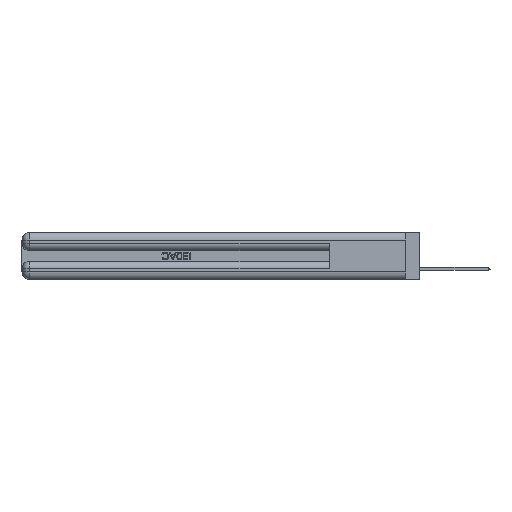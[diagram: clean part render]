
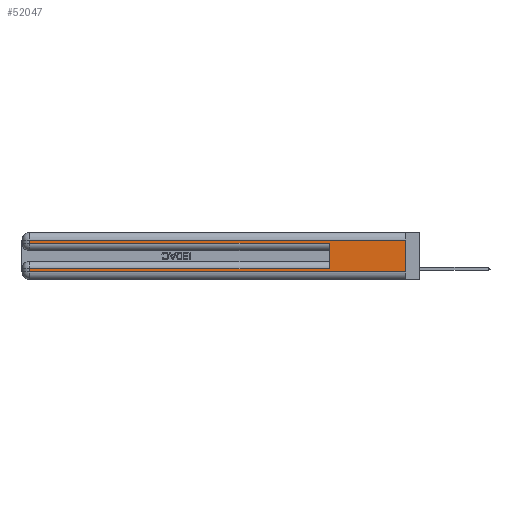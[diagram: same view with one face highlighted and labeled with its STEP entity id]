
A CAD part, left-side view. The second image highlights one B-rep face of the part: STEP entity #52047.
In plain terms, the highlighted planar face has unit normal (-1, 0, 0).
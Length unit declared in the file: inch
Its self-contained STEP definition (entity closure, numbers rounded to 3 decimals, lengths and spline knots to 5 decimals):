
#6 = CARTESIAN_POINT ( 'NONE',  ( 0., 0., 0.06 ) ) ;
#187 = CARTESIAN_POINT ( 'NONE',  ( 0., 0., 0.285 ) ) ;
#195 = ORIENTED_EDGE ( 'NONE', *, *, #5436, .T. ) ;
#637 = CARTESIAN_POINT ( 'NONE',  ( 0., 0., 0.31 ) ) ;
#955 = CARTESIAN_POINT ( 'NONE',  ( 0., 0., 0.06 ) ) ;
#1082 = VERTEX_POINT ( 'NONE', #637 ) ;
#1723 = LINE ( 'NONE', #17442, #22426 ) ;
#2922 = VECTOR ( 'NONE', #4155, 39.37008 ) ;
#3585 = CARTESIAN_POINT ( 'NONE',  ( 0., 0., 0.31 ) ) ;
#4155 = DIRECTION ( 'NONE',  ( 0., -1., 0. ) ) ;
#4736 = VECTOR ( 'NONE', #31438, 39.37008 ) ;
#4841 = LINE ( 'NONE', #187, #2922 ) ;
#5436 = EDGE_CURVE ( 'NONE', #20726, #36652, #41335, .T. ) ;
#6046 = DIRECTION ( 'NONE',  ( 0., 0., -1. ) ) ;
#6080 = DIRECTION ( 'NONE',  ( 0., 0., -1. ) ) ;
#6110 = ORIENTED_EDGE ( 'NONE', *, *, #36072, .T. ) ;
#6994 = ORIENTED_EDGE ( 'NONE', *, *, #25234, .T. ) ;
#8618 = DIRECTION ( 'NONE',  ( 0., 1., 0. ) ) ;
#9537 = LINE ( 'NONE', #36365, #23140 ) ;
#10032 = CARTESIAN_POINT ( 'NONE',  ( 0., 2.94, 0.285 ) ) ;
#10349 = CARTESIAN_POINT ( 'NONE',  ( 0., 2.94, 0.085 ) ) ;
#11581 = VERTEX_POINT ( 'NONE', #40566 ) ;
#12338 = EDGE_LOOP ( 'NONE', ( #43160, #6994, #46477, #6110, #37557, #43852, #195, #21215 ) ) ;
#13707 = VERTEX_POINT ( 'NONE', #14986 ) ;
#13824 = CARTESIAN_POINT ( 'NONE',  ( 0., 0., 0.37 ) ) ;
#14556 = CARTESIAN_POINT ( 'NONE',  ( 0., 0., 0.37 ) ) ;
#14986 = CARTESIAN_POINT ( 'NONE',  ( 0., 2.94, 0.31 ) ) ;
#14989 = CARTESIAN_POINT ( 'NONE',  ( 0., 0., 0.085 ) ) ;
#15681 = CARTESIAN_POINT ( 'NONE',  ( 0., 2.94, 0.06 ) ) ;
#17442 = CARTESIAN_POINT ( 'NONE',  ( 0., 0.6, 0.145 ) ) ;
#18283 = CARTESIAN_POINT ( 'NONE',  ( 0., 0.6, 0.085 ) ) ;
#20726 = VERTEX_POINT ( 'NONE', #10349 ) ;
#20862 = EDGE_CURVE ( 'NONE', #1082, #44634, #23156, .T. ) ;
#21215 = ORIENTED_EDGE ( 'NONE', *, *, #30833, .T. ) ;
#22426 = VECTOR ( 'NONE', #43666, 39.37008 ) ;
#23140 = VECTOR ( 'NONE', #44906, 39.37008 ) ;
#23156 = LINE ( 'NONE', #13824, #30892 ) ;
#25234 = EDGE_CURVE ( 'NONE', #1082, #13707, #48659, .T. ) ;
#26543 = DIRECTION ( 'NONE',  ( 1., 0., 0. ) ) ;
#26676 = VERTEX_POINT ( 'NONE', #18283 ) ;
#27069 = EDGE_CURVE ( 'NONE', #26676, #11581, #1723, .T. ) ;
#27201 = LINE ( 'NONE', #955, #38248 ) ;
#28112 = DIRECTION ( 'NONE',  ( 0., 0., -1. ) ) ;
#29643 = EDGE_CURVE ( 'NONE', #26676, #20726, #39682, .T. ) ;
#30833 = EDGE_CURVE ( 'NONE', #36652, #44634, #27201, .T. ) ;
#30892 = VECTOR ( 'NONE', #6046, 39.37008 ) ;
#31438 = DIRECTION ( 'NONE',  ( 0., 1., 0. ) ) ;
#32187 = VECTOR ( 'NONE', #28112, 39.37008 ) ;
#34499 = EDGE_CURVE ( 'NONE', #13707, #47899, #9537, .T. ) ;
#36072 = EDGE_CURVE ( 'NONE', #47899, #11581, #4841, .T. ) ;
#36365 = CARTESIAN_POINT ( 'NONE',  ( 0., 2.94, 0.37 ) ) ;
#36652 = VERTEX_POINT ( 'NONE', #15681 ) ;
#37557 = ORIENTED_EDGE ( 'NONE', *, *, #27069, .F. ) ;
#37659 = VECTOR ( 'NONE', #8618, 39.37008 ) ;
#38248 = VECTOR ( 'NONE', #47090, 39.37008 ) ;
#39611 = AXIS2_PLACEMENT_3D ( 'NONE', #14556, #26543, #6080 ) ;
#39682 = LINE ( 'NONE', #14989, #4736 ) ;
#39960 = FACE_OUTER_BOUND ( 'NONE', #12338, .T. ) ;
#40566 = CARTESIAN_POINT ( 'NONE',  ( 0., 0.6, 0.285 ) ) ;
#41335 = LINE ( 'NONE', #52340, #32187 ) ;
#43160 = ORIENTED_EDGE ( 'NONE', *, *, #20862, .F. ) ;
#43666 = DIRECTION ( 'NONE',  ( 0., 0., 1. ) ) ;
#43852 = ORIENTED_EDGE ( 'NONE', *, *, #29643, .T. ) ;
#44634 = VERTEX_POINT ( 'NONE', #6 ) ;
#44906 = DIRECTION ( 'NONE',  ( 0., 0., -1. ) ) ;
#46477 = ORIENTED_EDGE ( 'NONE', *, *, #34499, .T. ) ;
#47090 = DIRECTION ( 'NONE',  ( 0., -1., 0. ) ) ;
#47899 = VERTEX_POINT ( 'NONE', #10032 ) ;
#48659 = LINE ( 'NONE', #3585, #37659 ) ;
#51332 = PLANE ( 'NONE',  #39611 ) ;
#52047 = ADVANCED_FACE ( 'NONE', ( #39960 ), #51332, .F. ) ;
#52340 = CARTESIAN_POINT ( 'NONE',  ( 0., 2.94, 0.37 ) ) ;
